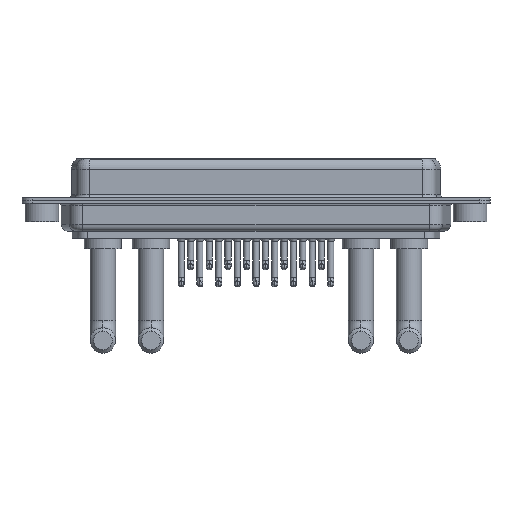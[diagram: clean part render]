
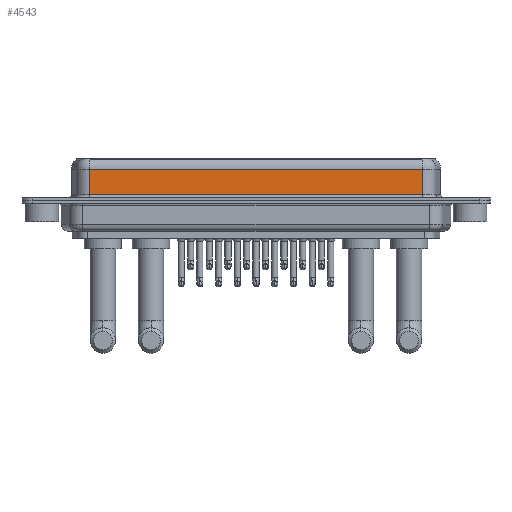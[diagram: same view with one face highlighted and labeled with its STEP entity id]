
A CAD part, front view. The second image highlights one B-rep face of the part: STEP entity #4543.
In plain terms, the highlighted planar face has unit normal (0, -1, 0).
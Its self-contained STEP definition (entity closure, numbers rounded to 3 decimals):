
#55 = VECTOR ( 'NONE', #11256, 1000. ) ;
#1040 = CARTESIAN_POINT ( 'NONE',  ( 7.038, -3.95, 6.4 ) ) ;
#1085 = EDGE_CURVE ( 'NONE', #10162, #17188, #16643, .T. ) ;
#2703 = DIRECTION ( 'NONE',  ( 0., 1., 0. ) ) ;
#2821 = DIRECTION ( 'NONE',  ( 0., 0., 1. ) ) ;
#4543 = ADVANCED_FACE ( 'NONE', ( #11932 ), #17492, .F. ) ;
#4771 = EDGE_CURVE ( 'NONE', #10408, #10162, #7688, .T. ) ;
#5870 = ORIENTED_EDGE ( 'NONE', *, *, #4771, .T. ) ;
#6206 = CARTESIAN_POINT ( 'NONE',  ( 7.038, -3.95, 0.9 ) ) ;
#6834 = AXIS2_PLACEMENT_3D ( 'NONE', #14528, #2703, #2821 ) ;
#6836 = CARTESIAN_POINT ( 'NONE',  ( 56.462, -3.95, 0.9 ) ) ;
#6849 = DIRECTION ( 'NONE',  ( 1., 0., 0. ) ) ;
#7170 = VERTEX_POINT ( 'NONE', #6836 ) ;
#7688 = LINE ( 'NONE', #10807, #55 ) ;
#8446 = EDGE_CURVE ( 'NONE', #10408, #7170, #16099, .T. ) ;
#9807 = EDGE_CURVE ( 'NONE', #17188, #7170, #13864, .T. ) ;
#10162 = VERTEX_POINT ( 'NONE', #19818 ) ;
#10408 = VERTEX_POINT ( 'NONE', #17489 ) ;
#10807 = CARTESIAN_POINT ( 'NONE',  ( 56.462, -3.95, 4.65 ) ) ;
#11256 = DIRECTION ( 'NONE',  ( -1., 0., 0. ) ) ;
#11932 = FACE_OUTER_BOUND ( 'NONE', #12245, .T. ) ;
#12245 = EDGE_LOOP ( 'NONE', ( #19446, #5870, #20973, #12723 ) ) ;
#12723 = ORIENTED_EDGE ( 'NONE', *, *, #9807, .T. ) ;
#13211 = DIRECTION ( 'NONE',  ( 0., 0., -1. ) ) ;
#13864 = LINE ( 'NONE', #17197, #16585 ) ;
#14000 = CARTESIAN_POINT ( 'NONE',  ( 56.462, -3.95, 6.4 ) ) ;
#14528 = CARTESIAN_POINT ( 'NONE',  ( 56.462, -3.95, 6.4 ) ) ;
#15488 = VECTOR ( 'NONE', #21064, 1000. ) ;
#16099 = LINE ( 'NONE', #14000, #15488 ) ;
#16585 = VECTOR ( 'NONE', #6849, 1000. ) ;
#16643 = LINE ( 'NONE', #1040, #16822 ) ;
#16822 = VECTOR ( 'NONE', #13211, 1000. ) ;
#17188 = VERTEX_POINT ( 'NONE', #6206 ) ;
#17197 = CARTESIAN_POINT ( 'NONE',  ( 56.462, -3.95, 0.9 ) ) ;
#17489 = CARTESIAN_POINT ( 'NONE',  ( 56.462, -3.95, 4.65 ) ) ;
#17492 = PLANE ( 'NONE',  #6834 ) ;
#19446 = ORIENTED_EDGE ( 'NONE', *, *, #8446, .F. ) ;
#19818 = CARTESIAN_POINT ( 'NONE',  ( 7.038, -3.95, 4.65 ) ) ;
#20973 = ORIENTED_EDGE ( 'NONE', *, *, #1085, .T. ) ;
#21064 = DIRECTION ( 'NONE',  ( 0., 0., -1. ) ) ;
